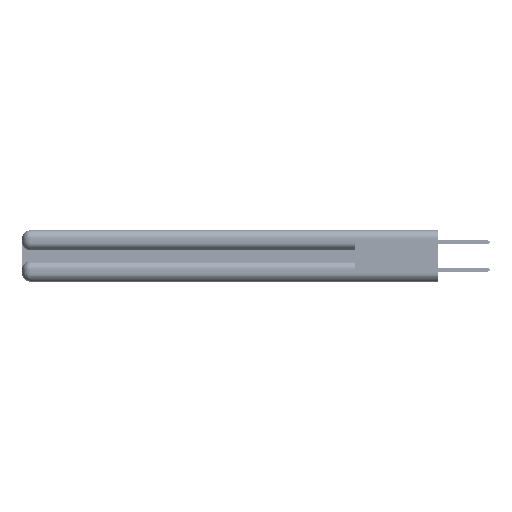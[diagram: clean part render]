
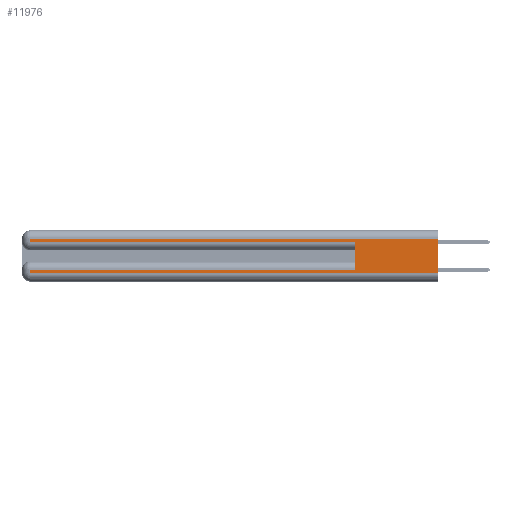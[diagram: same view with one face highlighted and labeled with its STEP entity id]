
A CAD part, left-side view. The second image highlights one B-rep face of the part: STEP entity #11976.
In plain terms, the highlighted planar face has unit normal (-1, 0, 0).
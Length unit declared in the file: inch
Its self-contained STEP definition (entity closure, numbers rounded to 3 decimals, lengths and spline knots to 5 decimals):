
#466 = CARTESIAN_POINT ( 'NONE',  ( 0., 0., 0.31 ) ) ;
#740 = DIRECTION ( 'NONE',  ( 1., 0., 0. ) ) ;
#1444 = CARTESIAN_POINT ( 'NONE',  ( 0., 0., 0.37 ) ) ;
#1785 = LINE ( 'NONE', #38459, #22367 ) ;
#3038 = CARTESIAN_POINT ( 'NONE',  ( 0., 2.94, 0.31 ) ) ;
#3154 = VERTEX_POINT ( 'NONE', #3038 ) ;
#5344 = DIRECTION ( 'NONE',  ( 0., 1., 0. ) ) ;
#5548 = EDGE_CURVE ( 'NONE', #3154, #31803, #1785, .T. ) ;
#6421 = LINE ( 'NONE', #43153, #37873 ) ;
#6629 = VECTOR ( 'NONE', #32286, 39.37008 ) ;
#7666 = CARTESIAN_POINT ( 'NONE',  ( 0., 0.6, 0.145 ) ) ;
#8832 = VERTEX_POINT ( 'NONE', #15785 ) ;
#10986 = VECTOR ( 'NONE', #17635, 39.37008 ) ;
#11976 = ADVANCED_FACE ( 'NONE', ( #53107 ), #49904, .F. ) ;
#12123 = EDGE_CURVE ( 'NONE', #25544, #8832, #37098, .T. ) ;
#12348 = ORIENTED_EDGE ( 'NONE', *, *, #19078, .T. ) ;
#12997 = CARTESIAN_POINT ( 'NONE',  ( 0., 0., 0.37 ) ) ;
#14423 = CARTESIAN_POINT ( 'NONE',  ( 0., 0.6, 0.085 ) ) ;
#14789 = ORIENTED_EDGE ( 'NONE', *, *, #24956, .T. ) ;
#14834 = VERTEX_POINT ( 'NONE', #41022 ) ;
#15785 = CARTESIAN_POINT ( 'NONE',  ( 0., 0., 0.06 ) ) ;
#17553 = CARTESIAN_POINT ( 'NONE',  ( 0., 0., 0.31 ) ) ;
#17635 = DIRECTION ( 'NONE',  ( 0., 0., -1. ) ) ;
#18108 = CARTESIAN_POINT ( 'NONE',  ( 0., 0., 0.085 ) ) ;
#18661 = VECTOR ( 'NONE', #46780, 39.37008 ) ;
#19078 = EDGE_CURVE ( 'NONE', #51013, #8832, #6421, .T. ) ;
#19308 = ORIENTED_EDGE ( 'NONE', *, *, #31375, .T. ) ;
#21991 = DIRECTION ( 'NONE',  ( 0., 0., -1. ) ) ;
#22367 = VECTOR ( 'NONE', #21991, 39.37008 ) ;
#22735 = DIRECTION ( 'NONE',  ( 0., -1., 0. ) ) ;
#24956 = EDGE_CURVE ( 'NONE', #31803, #28290, #45568, .T. ) ;
#25544 = VERTEX_POINT ( 'NONE', #466 ) ;
#28290 = VERTEX_POINT ( 'NONE', #31740 ) ;
#28512 = LINE ( 'NONE', #7666, #6629 ) ;
#28554 = DIRECTION ( 'NONE',  ( 0., -1., 0. ) ) ;
#28766 = EDGE_LOOP ( 'NONE', ( #31513, #50095, #43019, #14789, #40485, #19308, #29935, #12348 ) ) ;
#29502 = DIRECTION ( 'NONE',  ( 0., 0., -1. ) ) ;
#29935 = ORIENTED_EDGE ( 'NONE', *, *, #52363, .T. ) ;
#30057 = CARTESIAN_POINT ( 'NONE',  ( 0., 2.94, 0.37 ) ) ;
#30205 = DIRECTION ( 'NONE',  ( 0., 0., -1. ) ) ;
#31375 = EDGE_CURVE ( 'NONE', #47462, #14834, #50085, .T. ) ;
#31513 = ORIENTED_EDGE ( 'NONE', *, *, #12123, .F. ) ;
#31740 = CARTESIAN_POINT ( 'NONE',  ( 0., 0.6, 0.285 ) ) ;
#31803 = VERTEX_POINT ( 'NONE', #36930 ) ;
#32207 = CARTESIAN_POINT ( 'NONE',  ( 0., 2.94, 0.06 ) ) ;
#32286 = DIRECTION ( 'NONE',  ( 0., 0., 1. ) ) ;
#34726 = VECTOR ( 'NONE', #28554, 39.37008 ) ;
#35812 = VECTOR ( 'NONE', #5344, 39.37008 ) ;
#36930 = CARTESIAN_POINT ( 'NONE',  ( 0., 2.94, 0.285 ) ) ;
#37098 = LINE ( 'NONE', #1444, #46674 ) ;
#37873 = VECTOR ( 'NONE', #22735, 39.37008 ) ;
#38459 = CARTESIAN_POINT ( 'NONE',  ( 0., 2.94, 0.37 ) ) ;
#40485 = ORIENTED_EDGE ( 'NONE', *, *, #46464, .F. ) ;
#40725 = CARTESIAN_POINT ( 'NONE',  ( 0., 0., 0.285 ) ) ;
#41022 = CARTESIAN_POINT ( 'NONE',  ( 0., 2.94, 0.085 ) ) ;
#42433 = LINE ( 'NONE', #30057, #10986 ) ;
#43019 = ORIENTED_EDGE ( 'NONE', *, *, #5548, .T. ) ;
#43153 = CARTESIAN_POINT ( 'NONE',  ( 0., 0., 0.06 ) ) ;
#45129 = AXIS2_PLACEMENT_3D ( 'NONE', #12997, #740, #29502 ) ;
#45568 = LINE ( 'NONE', #40725, #34726 ) ;
#46464 = EDGE_CURVE ( 'NONE', #47462, #28290, #28512, .T. ) ;
#46668 = LINE ( 'NONE', #17553, #35812 ) ;
#46674 = VECTOR ( 'NONE', #30205, 39.37008 ) ;
#46780 = DIRECTION ( 'NONE',  ( 0., 1., 0. ) ) ;
#47462 = VERTEX_POINT ( 'NONE', #14423 ) ;
#49904 = PLANE ( 'NONE',  #45129 ) ;
#49941 = EDGE_CURVE ( 'NONE', #25544, #3154, #46668, .T. ) ;
#50085 = LINE ( 'NONE', #18108, #18661 ) ;
#50095 = ORIENTED_EDGE ( 'NONE', *, *, #49941, .T. ) ;
#51013 = VERTEX_POINT ( 'NONE', #32207 ) ;
#52363 = EDGE_CURVE ( 'NONE', #14834, #51013, #42433, .T. ) ;
#53107 = FACE_OUTER_BOUND ( 'NONE', #28766, .T. ) ;
